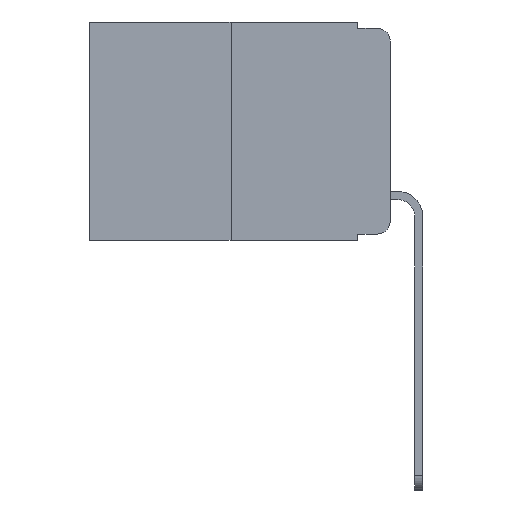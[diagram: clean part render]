
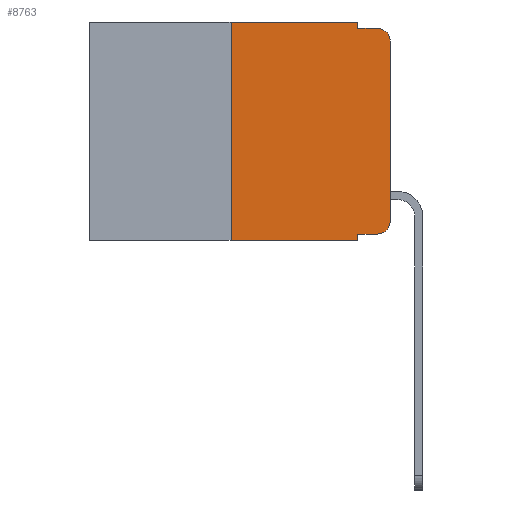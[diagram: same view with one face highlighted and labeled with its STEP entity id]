
A CAD part, left-side view. The second image highlights one B-rep face of the part: STEP entity #8763.
In plain terms, the highlighted planar face has unit normal (-1, 0, 0).
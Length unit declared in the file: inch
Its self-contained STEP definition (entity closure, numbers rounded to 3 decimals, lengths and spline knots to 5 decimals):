
#260 = CARTESIAN_POINT ( 'NONE',  ( 0., 0.25, 0. ) ) ;
#439 = ORIENTED_EDGE ( 'NONE', *, *, #8830, .T. ) ;
#565 = DIRECTION ( 'NONE',  ( 0., -1., 0. ) ) ;
#692 = AXIS2_PLACEMENT_3D ( 'NONE', #10343, #4243, #11367 ) ;
#1229 = VERTEX_POINT ( 'NONE', #12831 ) ;
#1312 = CARTESIAN_POINT ( 'NONE',  ( 0., 0.051, -0.343 ) ) ;
#1477 = VERTEX_POINT ( 'NONE', #11743 ) ;
#1564 = CARTESIAN_POINT ( 'NONE',  ( 0., 0.02, -0.01 ) ) ;
#2632 = ORIENTED_EDGE ( 'NONE', *, *, #13400, .T. ) ;
#2666 = DIRECTION ( 'NONE',  ( 0., 0., -1. ) ) ;
#2909 = PLANE ( 'NONE',  #4444 ) ;
#3112 = EDGE_CURVE ( 'NONE', #5545, #7238, #7276, .T. ) ;
#3113 = ORIENTED_EDGE ( 'NONE', *, *, #3112, .F. ) ;
#3159 = CARTESIAN_POINT ( 'NONE',  ( 0., 0.25, -0.343 ) ) ;
#3409 = ORIENTED_EDGE ( 'NONE', *, *, #6161, .F. ) ;
#3586 = DIRECTION ( 'NONE',  ( 0., 0., 1. ) ) ;
#3863 = VECTOR ( 'NONE', #3586, 39.37008 ) ;
#3896 = VERTEX_POINT ( 'NONE', #1312 ) ;
#4027 = VERTEX_POINT ( 'NONE', #1564 ) ;
#4179 = LINE ( 'NONE', #12761, #3863 ) ;
#4243 = DIRECTION ( 'NONE',  ( -1., 0., 0. ) ) ;
#4290 = CARTESIAN_POINT ( 'NONE',  ( 0., 0.051, 0. ) ) ;
#4304 = LINE ( 'NONE', #13259, #9409 ) ;
#4444 = AXIS2_PLACEMENT_3D ( 'NONE', #11097, #13179, #7055 ) ;
#4689 = VECTOR ( 'NONE', #2666, 39.37008 ) ;
#4966 = CARTESIAN_POINT ( 'NONE',  ( 0., 0.051, -0.333 ) ) ;
#5042 = VERTEX_POINT ( 'NONE', #7499 ) ;
#5235 = EDGE_CURVE ( 'NONE', #7238, #4027, #12351, .T. ) ;
#5544 = CIRCLE ( 'NONE', #11979, 0.02 ) ;
#5545 = VERTEX_POINT ( 'NONE', #12105 ) ;
#5718 = ORIENTED_EDGE ( 'NONE', *, *, #5235, .F. ) ;
#5748 = EDGE_CURVE ( 'NONE', #7687, #1229, #10564, .T. ) ;
#5889 = LINE ( 'NONE', #260, #8567 ) ;
#5904 = VECTOR ( 'NONE', #565, 39.37008 ) ;
#5944 = CARTESIAN_POINT ( 'NONE',  ( 0., 0.473, 0. ) ) ;
#6077 = CARTESIAN_POINT ( 'NONE',  ( 0., 0.051, -0.01 ) ) ;
#6161 = EDGE_CURVE ( 'NONE', #1477, #3896, #12487, .T. ) ;
#6446 = CARTESIAN_POINT ( 'NONE',  ( 0., 0.02, -0.03 ) ) ;
#6696 = CARTESIAN_POINT ( 'NONE',  ( 0., 0.02, -0.333 ) ) ;
#6729 = DIRECTION ( 'NONE',  ( 0., 0., 1. ) ) ;
#6734 = DIRECTION ( 'NONE',  ( 0., -1., 0. ) ) ;
#6766 = LINE ( 'NONE', #5944, #11852 ) ;
#6797 = CARTESIAN_POINT ( 'NONE',  ( 0., 0.25, 0. ) ) ;
#7055 = DIRECTION ( 'NONE',  ( 0., 0., -1. ) ) ;
#7120 = EDGE_CURVE ( 'NONE', #9428, #5545, #6766, .T. ) ;
#7238 = VERTEX_POINT ( 'NONE', #6077 ) ;
#7276 = LINE ( 'NONE', #4290, #12072 ) ;
#7443 = DIRECTION ( 'NONE',  ( 0., 0., -1. ) ) ;
#7499 = CARTESIAN_POINT ( 'NONE',  ( 0., 0., -0.03 ) ) ;
#7580 = ORIENTED_EDGE ( 'NONE', *, *, #10479, .T. ) ;
#7687 = VERTEX_POINT ( 'NONE', #6696 ) ;
#8567 = VECTOR ( 'NONE', #6729, 39.37008 ) ;
#8763 = ADVANCED_FACE ( 'NONE', ( #12779 ), #2909, .F. ) ;
#8829 = CARTESIAN_POINT ( 'NONE',  ( 0., 0.051, 0. ) ) ;
#8830 = EDGE_CURVE ( 'NONE', #9850, #3896, #4304, .T. ) ;
#9016 = ORIENTED_EDGE ( 'NONE', *, *, #7120, .F. ) ;
#9182 = DIRECTION ( 'NONE',  ( 0., -1., 0. ) ) ;
#9301 = VECTOR ( 'NONE', #6734, 39.37008 ) ;
#9409 = VECTOR ( 'NONE', #9182, 39.37008 ) ;
#9428 = VERTEX_POINT ( 'NONE', #6797 ) ;
#9831 = ORIENTED_EDGE ( 'NONE', *, *, #11337, .T. ) ;
#9850 = VERTEX_POINT ( 'NONE', #3159 ) ;
#10136 = ORIENTED_EDGE ( 'NONE', *, *, #5748, .T. ) ;
#10343 = CARTESIAN_POINT ( 'NONE',  ( 0., 0.02, -0.313 ) ) ;
#10479 = EDGE_CURVE ( 'NONE', #1477, #7687, #11942, .T. ) ;
#10564 = CIRCLE ( 'NONE', #692, 0.02 ) ;
#10913 = EDGE_CURVE ( 'NONE', #9850, #9428, #5889, .T. ) ;
#10934 = ORIENTED_EDGE ( 'NONE', *, *, #10913, .F. ) ;
#11097 = CARTESIAN_POINT ( 'NONE',  ( 0., 0.473, 0. ) ) ;
#11337 = EDGE_CURVE ( 'NONE', #5042, #4027, #5544, .T. ) ;
#11367 = DIRECTION ( 'NONE',  ( 0., 0., -1. ) ) ;
#11423 = DIRECTION ( 'NONE',  ( 0., 0., -1. ) ) ;
#11743 = CARTESIAN_POINT ( 'NONE',  ( 0., 0.051, -0.333 ) ) ;
#11802 = CARTESIAN_POINT ( 'NONE',  ( 0., 0.051, -0.01 ) ) ;
#11852 = VECTOR ( 'NONE', #12029, 39.37008 ) ;
#11942 = LINE ( 'NONE', #4966, #5904 ) ;
#11979 = AXIS2_PLACEMENT_3D ( 'NONE', #6446, #13563, #7443 ) ;
#12029 = DIRECTION ( 'NONE',  ( 0., -1., 0. ) ) ;
#12072 = VECTOR ( 'NONE', #11423, 39.37008 ) ;
#12105 = CARTESIAN_POINT ( 'NONE',  ( 0., 0.051, 0. ) ) ;
#12160 = EDGE_LOOP ( 'NONE', ( #2632, #9831, #5718, #3113, #9016, #10934, #439, #3409, #7580, #10136 ) ) ;
#12351 = LINE ( 'NONE', #11802, #9301 ) ;
#12487 = LINE ( 'NONE', #8829, #4689 ) ;
#12761 = CARTESIAN_POINT ( 'NONE',  ( 0., 0., 0. ) ) ;
#12779 = FACE_OUTER_BOUND ( 'NONE', #12160, .T. ) ;
#12831 = CARTESIAN_POINT ( 'NONE',  ( 0., 0., -0.313 ) ) ;
#13179 = DIRECTION ( 'NONE',  ( 1., 0., 0. ) ) ;
#13259 = CARTESIAN_POINT ( 'NONE',  ( 0., 0.473, -0.343 ) ) ;
#13400 = EDGE_CURVE ( 'NONE', #1229, #5042, #4179, .T. ) ;
#13563 = DIRECTION ( 'NONE',  ( -1., 0., 0. ) ) ;
